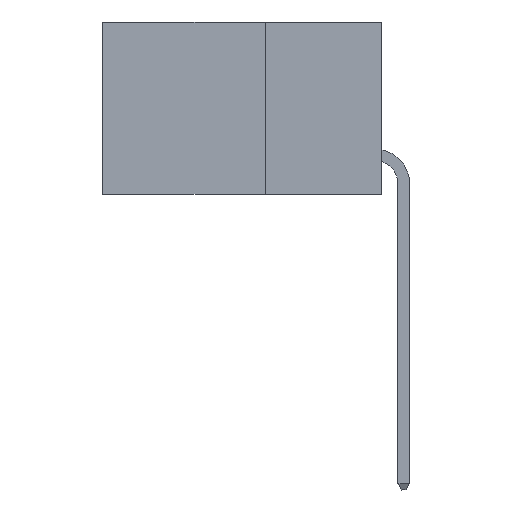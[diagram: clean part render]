
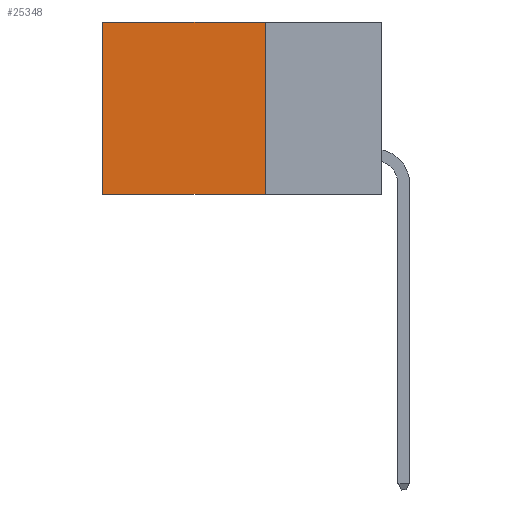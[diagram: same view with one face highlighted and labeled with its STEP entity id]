
A CAD part, left-side view. The second image highlights one B-rep face of the part: STEP entity #25348.
In plain terms, the highlighted planar face has unit normal (-1, 0, 0).
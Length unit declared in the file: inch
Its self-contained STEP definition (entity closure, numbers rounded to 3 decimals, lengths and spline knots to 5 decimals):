
#858 = CARTESIAN_POINT ( 'NONE',  ( 0.2875, 0.25, 0. ) ) ;
#974 = DIRECTION ( 'NONE',  ( 0., 1., 0. ) ) ;
#3205 = DIRECTION ( 'NONE',  ( 0., 0., -1. ) ) ;
#3528 = LINE ( 'NONE', #22935, #8222 ) ;
#3535 = VECTOR ( 'NONE', #974, 39.37008 ) ;
#4021 = VERTEX_POINT ( 'NONE', #9111 ) ;
#5168 = EDGE_CURVE ( 'NONE', #22560, #20709, #20651, .T. ) ;
#5736 = FACE_OUTER_BOUND ( 'NONE', #11889, .T. ) ;
#7262 = EDGE_CURVE ( 'NONE', #17017, #22560, #9707, .T. ) ;
#7941 = ORIENTED_EDGE ( 'NONE', *, *, #7262, .T. ) ;
#8014 = CARTESIAN_POINT ( 'NONE',  ( 0.2875, 0.25, 0. ) ) ;
#8222 = VECTOR ( 'NONE', #25229, 39.37008 ) ;
#9111 = CARTESIAN_POINT ( 'NONE',  ( 0.2875, 0.25, -0.37 ) ) ;
#9233 = AXIS2_PLACEMENT_3D ( 'NONE', #858, #17099, #3205 ) ;
#9318 = VECTOR ( 'NONE', #15039, 39.37008 ) ;
#9707 = LINE ( 'NONE', #28570, #3535 ) ;
#11889 = EDGE_LOOP ( 'NONE', ( #23644, #23696, #12650, #7941 ) ) ;
#12650 = ORIENTED_EDGE ( 'NONE', *, *, #19019, .F. ) ;
#12835 = EDGE_CURVE ( 'NONE', #4021, #20709, #3528, .T. ) ;
#13796 = CARTESIAN_POINT ( 'NONE',  ( 0.2875, 0.6, 0. ) ) ;
#15039 = DIRECTION ( 'NONE',  ( 0., 0., -1. ) ) ;
#15270 = VECTOR ( 'NONE', #20460, 39.37008 ) ;
#17017 = VERTEX_POINT ( 'NONE', #19356 ) ;
#17099 = DIRECTION ( 'NONE',  ( 1., 0., 0. ) ) ;
#18106 = CARTESIAN_POINT ( 'NONE',  ( 0.2875, 0.6, -0.37 ) ) ;
#19019 = EDGE_CURVE ( 'NONE', #17017, #4021, #27667, .T. ) ;
#19356 = CARTESIAN_POINT ( 'NONE',  ( 0.2875, 0.25, 0. ) ) ;
#20460 = DIRECTION ( 'NONE',  ( 0., 0., -1. ) ) ;
#20547 = CARTESIAN_POINT ( 'NONE',  ( 0.2875, 0.6, 0. ) ) ;
#20651 = LINE ( 'NONE', #20547, #15270 ) ;
#20709 = VERTEX_POINT ( 'NONE', #18106 ) ;
#22560 = VERTEX_POINT ( 'NONE', #13796 ) ;
#22935 = CARTESIAN_POINT ( 'NONE',  ( 0.2875, 0.25, -0.37 ) ) ;
#23644 = ORIENTED_EDGE ( 'NONE', *, *, #5168, .T. ) ;
#23696 = ORIENTED_EDGE ( 'NONE', *, *, #12835, .F. ) ;
#23910 = PLANE ( 'NONE',  #9233 ) ;
#25229 = DIRECTION ( 'NONE',  ( 0., 1., 0. ) ) ;
#25348 = ADVANCED_FACE ( 'NONE', ( #5736 ), #23910, .F. ) ;
#27667 = LINE ( 'NONE', #8014, #9318 ) ;
#28570 = CARTESIAN_POINT ( 'NONE',  ( 0.2875, 0.25, 0. ) ) ;
